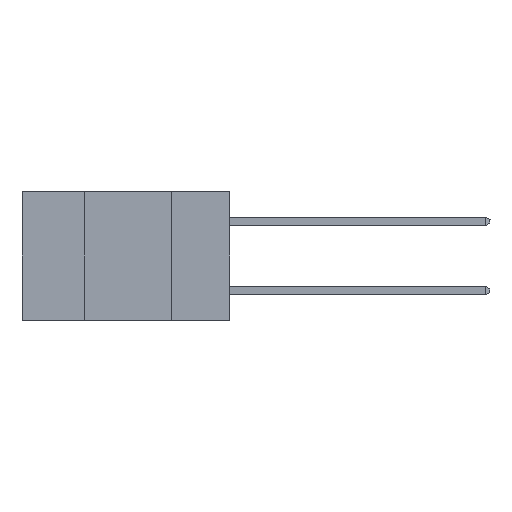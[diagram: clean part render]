
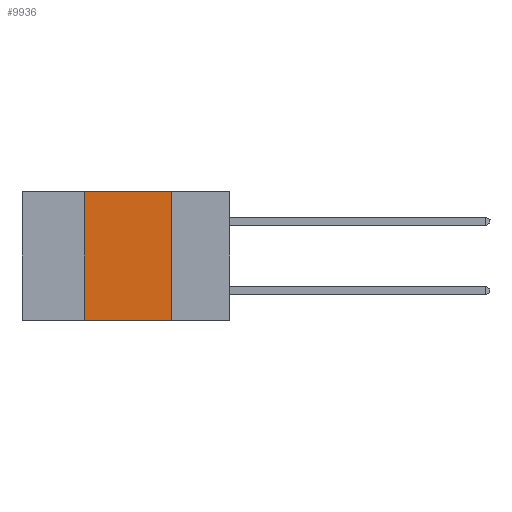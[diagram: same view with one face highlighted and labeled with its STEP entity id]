
A CAD part, left-side view. The second image highlights one B-rep face of the part: STEP entity #9936.
In plain terms, the highlighted planar face has unit normal (-1, 0, 0).
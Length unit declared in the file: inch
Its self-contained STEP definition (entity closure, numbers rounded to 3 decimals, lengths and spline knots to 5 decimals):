
#1187 = CARTESIAN_POINT ( 'NONE',  ( 0., 0.6, 0. ) ) ;
#1569 = VERTEX_POINT ( 'NONE', #1773 ) ;
#1773 = CARTESIAN_POINT ( 'NONE',  ( 0., 0.42, -0.37 ) ) ;
#1905 = LINE ( 'NONE', #14522, #7680 ) ;
#2781 = VECTOR ( 'NONE', #7353, 39.37008 ) ;
#3348 = CARTESIAN_POINT ( 'NONE',  ( 0., 0.17, -0.37 ) ) ;
#3642 = CARTESIAN_POINT ( 'NONE',  ( 0., 0.6, 0. ) ) ;
#3981 = VERTEX_POINT ( 'NONE', #3348 ) ;
#5014 = CARTESIAN_POINT ( 'NONE',  ( 0., 0.6, -0.37 ) ) ;
#5053 = FACE_OUTER_BOUND ( 'NONE', #18447, .T. ) ;
#5156 = DIRECTION ( 'NONE',  ( 0., 0., -1. ) ) ;
#5536 = VERTEX_POINT ( 'NONE', #19235 ) ;
#5918 = LINE ( 'NONE', #1187, #2781 ) ;
#5969 = EDGE_CURVE ( 'NONE', #1569, #3981, #9855, .T. ) ;
#6031 = LINE ( 'NONE', #9432, #17296 ) ;
#7137 = CARTESIAN_POINT ( 'NONE',  ( 0., 0.42, 0. ) ) ;
#7353 = DIRECTION ( 'NONE',  ( 0., -1., 0. ) ) ;
#7680 = VECTOR ( 'NONE', #8052, 39.37008 ) ;
#8052 = DIRECTION ( 'NONE',  ( 0., 0., -1. ) ) ;
#8965 = EDGE_CURVE ( 'NONE', #1569, #19263, #6031, .T. ) ;
#9432 = CARTESIAN_POINT ( 'NONE',  ( 0., 0.42, -0.37 ) ) ;
#9681 = ORIENTED_EDGE ( 'NONE', *, *, #5969, .T. ) ;
#9748 = DIRECTION ( 'NONE',  ( 0., -1., 0. ) ) ;
#9855 = LINE ( 'NONE', #5014, #14703 ) ;
#9936 = ADVANCED_FACE ( 'NONE', ( #5053 ), #12854, .F. ) ;
#12769 = ORIENTED_EDGE ( 'NONE', *, *, #8965, .F. ) ;
#12854 = PLANE ( 'NONE',  #17936 ) ;
#13592 = ORIENTED_EDGE ( 'NONE', *, *, #15681, .F. ) ;
#14522 = CARTESIAN_POINT ( 'NONE',  ( 0., 0.17, -0.37 ) ) ;
#14703 = VECTOR ( 'NONE', #9748, 39.37008 ) ;
#14889 = ORIENTED_EDGE ( 'NONE', *, *, #19266, .F. ) ;
#15681 = EDGE_CURVE ( 'NONE', #5536, #3981, #1905, .T. ) ;
#16870 = DIRECTION ( 'NONE',  ( 0., 0., 1. ) ) ;
#17296 = VECTOR ( 'NONE', #16870, 39.37008 ) ;
#17936 = AXIS2_PLACEMENT_3D ( 'NONE', #3642, #19069, #5156 ) ;
#18447 = EDGE_LOOP ( 'NONE', ( #13592, #14889, #12769, #9681 ) ) ;
#19069 = DIRECTION ( 'NONE',  ( 1., 0., 0. ) ) ;
#19235 = CARTESIAN_POINT ( 'NONE',  ( 0., 0.17, 0. ) ) ;
#19263 = VERTEX_POINT ( 'NONE', #7137 ) ;
#19266 = EDGE_CURVE ( 'NONE', #19263, #5536, #5918, .T. ) ;
